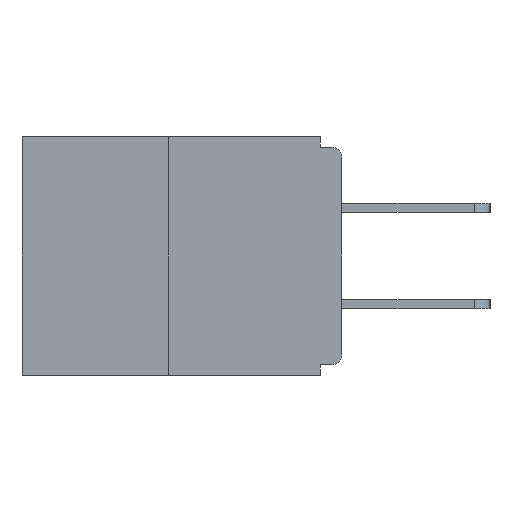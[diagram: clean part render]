
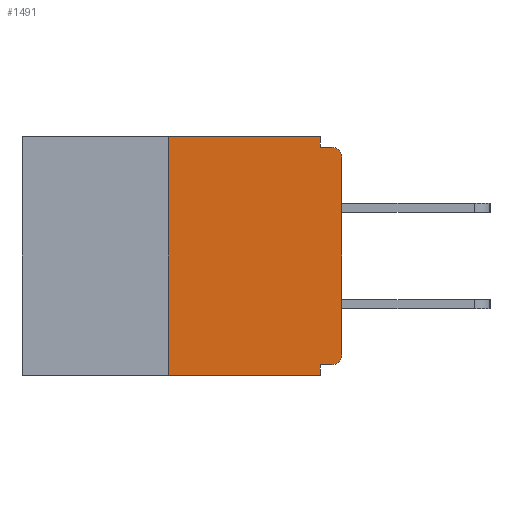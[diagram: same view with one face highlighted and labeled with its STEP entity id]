
A CAD part, left-side view. The second image highlights one B-rep face of the part: STEP entity #1491.
In plain terms, the highlighted planar face has unit normal (-1, 0, 0).
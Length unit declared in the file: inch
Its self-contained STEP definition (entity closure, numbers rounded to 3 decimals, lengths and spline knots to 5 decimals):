
#9 = ORIENTED_EDGE ( 'NONE', *, *, #2341, .F. ) ;
#265 = EDGE_CURVE ( 'NONE', #8932, #4390, #6730, .T. ) ;
#366 = EDGE_CURVE ( 'NONE', #8761, #4568, #2960, .T. ) ;
#1050 = VERTEX_POINT ( 'NONE', #10609 ) ;
#1173 = ORIENTED_EDGE ( 'NONE', *, *, #366, .F. ) ;
#1241 = CIRCLE ( 'NONE', #6238, 0.015 ) ;
#1491 = ADVANCED_FACE ( 'NONE', ( #6690 ), #5200, .F. ) ;
#1559 = LINE ( 'NONE', #3817, #10131 ) ;
#1763 = DIRECTION ( 'NONE',  ( -1., 0., 0. ) ) ;
#1971 = DIRECTION ( 'NONE',  ( -1., 0., 0. ) ) ;
#2000 = VERTEX_POINT ( 'NONE', #10686 ) ;
#2308 = CARTESIAN_POINT ( 'NONE',  ( 0., 0.031, 0. ) ) ;
#2341 = EDGE_CURVE ( 'NONE', #7189, #8761, #1559, .T. ) ;
#2390 = CARTESIAN_POINT ( 'NONE',  ( 0., 0.46, 0. ) ) ;
#2914 = AXIS2_PLACEMENT_3D ( 'NONE', #2390, #4255, #11295 ) ;
#2960 = LINE ( 'NONE', #8622, #11731 ) ;
#2975 = ORIENTED_EDGE ( 'NONE', *, *, #6458, .T. ) ;
#3109 = ORIENTED_EDGE ( 'NONE', *, *, #4591, .F. ) ;
#3213 = LINE ( 'NONE', #8738, #9496 ) ;
#3294 = ORIENTED_EDGE ( 'NONE', *, *, #265, .F. ) ;
#3817 = CARTESIAN_POINT ( 'NONE',  ( 0., 0.25, 0. ) ) ;
#4255 = DIRECTION ( 'NONE',  ( 1., 0., 0. ) ) ;
#4390 = VERTEX_POINT ( 'NONE', #5272 ) ;
#4568 = VERTEX_POINT ( 'NONE', #6653 ) ;
#4579 = CARTESIAN_POINT ( 'NONE',  ( 0., 0.015, -0.313 ) ) ;
#4591 = EDGE_CURVE ( 'NONE', #4568, #6976, #6249, .T. ) ;
#4622 = DIRECTION ( 'NONE',  ( 0., 0., -1. ) ) ;
#4726 = LINE ( 'NONE', #6792, #5191 ) ;
#4812 = ORIENTED_EDGE ( 'NONE', *, *, #9546, .T. ) ;
#4869 = ORIENTED_EDGE ( 'NONE', *, *, #7127, .T. ) ;
#5191 = VECTOR ( 'NONE', #6873, 39.37008 ) ;
#5200 = PLANE ( 'NONE',  #2914 ) ;
#5272 = CARTESIAN_POINT ( 'NONE',  ( 0., 0.031, -0.343 ) ) ;
#5329 = LINE ( 'NONE', #6629, #9908 ) ;
#5415 = LINE ( 'NONE', #7847, #7777 ) ;
#5612 = VECTOR ( 'NONE', #8656, 39.37008 ) ;
#5861 = DIRECTION ( 'NONE',  ( 0., 0., 1. ) ) ;
#6238 = AXIS2_PLACEMENT_3D ( 'NONE', #4579, #1763, #4622 ) ;
#6249 = LINE ( 'NONE', #2308, #5612 ) ;
#6417 = EDGE_CURVE ( 'NONE', #2000, #8932, #5415, .T. ) ;
#6458 = EDGE_CURVE ( 'NONE', #1050, #12363, #9999, .T. ) ;
#6629 = CARTESIAN_POINT ( 'NONE',  ( 0., 0.46, -0.343 ) ) ;
#6653 = CARTESIAN_POINT ( 'NONE',  ( 0., 0.031, 0. ) ) ;
#6667 = VERTEX_POINT ( 'NONE', #6968 ) ;
#6690 = FACE_OUTER_BOUND ( 'NONE', #7452, .T. ) ;
#6730 = LINE ( 'NONE', #8982, #11749 ) ;
#6792 = CARTESIAN_POINT ( 'NONE',  ( 0., 0., -0.015 ) ) ;
#6873 = DIRECTION ( 'NONE',  ( 0., -1., 0. ) ) ;
#6933 = DIRECTION ( 'NONE',  ( 0., 1., 0. ) ) ;
#6937 = EDGE_CURVE ( 'NONE', #6667, #1050, #3213, .T. ) ;
#6968 = CARTESIAN_POINT ( 'NONE',  ( 0., 0., -0.313 ) ) ;
#6976 = VERTEX_POINT ( 'NONE', #11945 ) ;
#7127 = EDGE_CURVE ( 'NONE', #2000, #6667, #1241, .T. ) ;
#7189 = VERTEX_POINT ( 'NONE', #9730 ) ;
#7452 = EDGE_LOOP ( 'NONE', ( #1173, #9, #4812, #3294, #8426, #4869, #8884, #2975, #9924, #3109 ) ) ;
#7530 = DIRECTION ( 'NONE',  ( 0., -1., 0. ) ) ;
#7777 = VECTOR ( 'NONE', #6933, 39.37008 ) ;
#7847 = CARTESIAN_POINT ( 'NONE',  ( 0., 0., -0.328 ) ) ;
#8426 = ORIENTED_EDGE ( 'NONE', *, *, #6417, .F. ) ;
#8622 = CARTESIAN_POINT ( 'NONE',  ( 0., 0.46, 0. ) ) ;
#8656 = DIRECTION ( 'NONE',  ( 0., 0., -1. ) ) ;
#8738 = CARTESIAN_POINT ( 'NONE',  ( 0., 0., 0. ) ) ;
#8761 = VERTEX_POINT ( 'NONE', #11810 ) ;
#8841 = DIRECTION ( 'NONE',  ( 0., 0., -1. ) ) ;
#8854 = DIRECTION ( 'NONE',  ( 0., 0., 1. ) ) ;
#8884 = ORIENTED_EDGE ( 'NONE', *, *, #6937, .T. ) ;
#8906 = EDGE_CURVE ( 'NONE', #6976, #12363, #4726, .T. ) ;
#8932 = VERTEX_POINT ( 'NONE', #12780 ) ;
#8982 = CARTESIAN_POINT ( 'NONE',  ( 0., 0.031, -0.343 ) ) ;
#9113 = DIRECTION ( 'NONE',  ( 0., 0., -1. ) ) ;
#9496 = VECTOR ( 'NONE', #5861, 39.37008 ) ;
#9546 = EDGE_CURVE ( 'NONE', #7189, #4390, #5329, .T. ) ;
#9730 = CARTESIAN_POINT ( 'NONE',  ( 0., 0.25, -0.343 ) ) ;
#9908 = VECTOR ( 'NONE', #7530, 39.37008 ) ;
#9917 = CARTESIAN_POINT ( 'NONE',  ( 0., 0.015, -0.03 ) ) ;
#9924 = ORIENTED_EDGE ( 'NONE', *, *, #8906, .F. ) ;
#9999 = CIRCLE ( 'NONE', #12609, 0.015 ) ;
#10131 = VECTOR ( 'NONE', #8854, 39.37008 ) ;
#10166 = CARTESIAN_POINT ( 'NONE',  ( 0., 0.015, -0.015 ) ) ;
#10609 = CARTESIAN_POINT ( 'NONE',  ( 0., 0., -0.03 ) ) ;
#10686 = CARTESIAN_POINT ( 'NONE',  ( 0., 0.015, -0.328 ) ) ;
#10775 = DIRECTION ( 'NONE',  ( 0., -1., 0. ) ) ;
#11295 = DIRECTION ( 'NONE',  ( 0., 0., -1. ) ) ;
#11731 = VECTOR ( 'NONE', #10775, 39.37008 ) ;
#11749 = VECTOR ( 'NONE', #9113, 39.37008 ) ;
#11810 = CARTESIAN_POINT ( 'NONE',  ( 0., 0.25, 0. ) ) ;
#11945 = CARTESIAN_POINT ( 'NONE',  ( 0., 0.031, -0.015 ) ) ;
#12363 = VERTEX_POINT ( 'NONE', #10166 ) ;
#12609 = AXIS2_PLACEMENT_3D ( 'NONE', #9917, #1971, #8841 ) ;
#12780 = CARTESIAN_POINT ( 'NONE',  ( 0., 0.031, -0.328 ) ) ;
